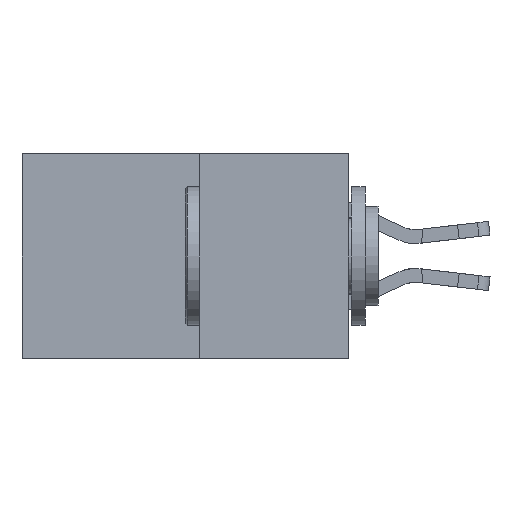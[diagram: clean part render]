
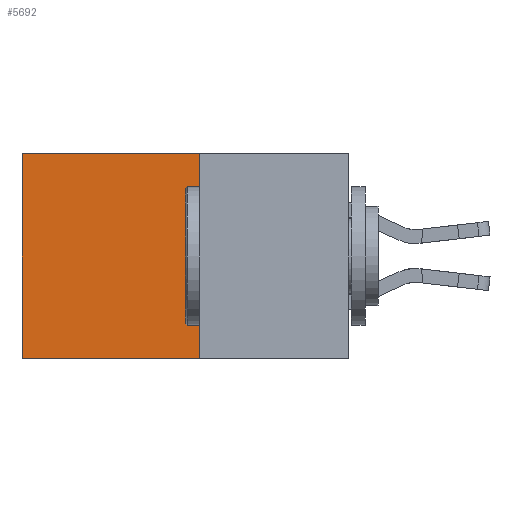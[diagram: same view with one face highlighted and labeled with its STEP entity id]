
A CAD part, left-side view. The second image highlights one B-rep face of the part: STEP entity #5692.
In plain terms, the highlighted planar face has unit normal (-1, 0, 0).
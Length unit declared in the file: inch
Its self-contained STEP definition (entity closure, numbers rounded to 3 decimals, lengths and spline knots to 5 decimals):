
#490 = ORIENTED_EDGE ( 'NONE', *, *, #3087, .T. ) ;
#864 = DIRECTION ( 'NONE',  ( 0., 0., -1. ) ) ;
#1040 = EDGE_CURVE ( 'NONE', #2628, #16681, #5359, .T. ) ;
#2305 = LINE ( 'NONE', #12895, #12979 ) ;
#2439 = CARTESIAN_POINT ( 'NONE',  ( 0.277, 0.27, 0. ) ) ;
#2628 = VERTEX_POINT ( 'NONE', #5415 ) ;
#3087 = EDGE_CURVE ( 'NONE', #9981, #16681, #4651, .T. ) ;
#3125 = DIRECTION ( 'NONE',  ( 0., 1., 0. ) ) ;
#4404 = ORIENTED_EDGE ( 'NONE', *, *, #1040, .F. ) ;
#4470 = DIRECTION ( 'NONE',  ( 0., 1., 0. ) ) ;
#4651 = LINE ( 'NONE', #12154, #14677 ) ;
#5359 = LINE ( 'NONE', #10289, #20069 ) ;
#5406 = PLANE ( 'NONE',  #6012 ) ;
#5415 = CARTESIAN_POINT ( 'NONE',  ( 0.277, 0.27, -0.37 ) ) ;
#5692 = ADVANCED_FACE ( 'NONE', ( #23560 ), #5406, .F. ) ;
#6012 = AXIS2_PLACEMENT_3D ( 'NONE', #13344, #19397, #7424 ) ;
#6582 = ORIENTED_EDGE ( 'NONE', *, *, #10410, .F. ) ;
#6950 = CARTESIAN_POINT ( 'NONE',  ( 0.277, 0.59, -0.37 ) ) ;
#7424 = DIRECTION ( 'NONE',  ( 0., 0., -1. ) ) ;
#9981 = VERTEX_POINT ( 'NONE', #12671 ) ;
#10289 = CARTESIAN_POINT ( 'NONE',  ( 0.277, 0.27, -0.37 ) ) ;
#10410 = EDGE_CURVE ( 'NONE', #10960, #2628, #2305, .T. ) ;
#10960 = VERTEX_POINT ( 'NONE', #14447 ) ;
#12154 = CARTESIAN_POINT ( 'NONE',  ( 0.277, 0.59, -0.37 ) ) ;
#12671 = CARTESIAN_POINT ( 'NONE',  ( 0.277, 0.59, 0. ) ) ;
#12895 = CARTESIAN_POINT ( 'NONE',  ( 0.277, 0.27, -0.37 ) ) ;
#12979 = VECTOR ( 'NONE', #864, 39.37008 ) ;
#13344 = CARTESIAN_POINT ( 'NONE',  ( 0.277, 0.27, -0.37 ) ) ;
#14263 = LINE ( 'NONE', #2439, #24221 ) ;
#14447 = CARTESIAN_POINT ( 'NONE',  ( 0.277, 0.27, 0. ) ) ;
#14677 = VECTOR ( 'NONE', #18814, 39.37008 ) ;
#15298 = ORIENTED_EDGE ( 'NONE', *, *, #16213, .T. ) ;
#16213 = EDGE_CURVE ( 'NONE', #10960, #9981, #14263, .T. ) ;
#16681 = VERTEX_POINT ( 'NONE', #6950 ) ;
#18657 = EDGE_LOOP ( 'NONE', ( #490, #4404, #6582, #15298 ) ) ;
#18814 = DIRECTION ( 'NONE',  ( 0., 0., -1. ) ) ;
#19397 = DIRECTION ( 'NONE',  ( 1., 0., 0. ) ) ;
#20069 = VECTOR ( 'NONE', #3125, 39.37008 ) ;
#23560 = FACE_OUTER_BOUND ( 'NONE', #18657, .T. ) ;
#24221 = VECTOR ( 'NONE', #4470, 39.37008 ) ;
